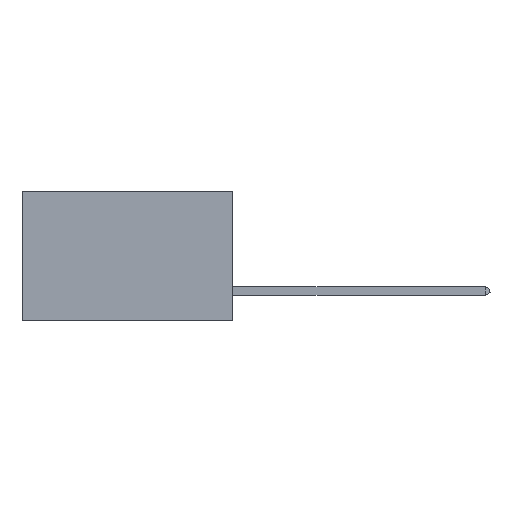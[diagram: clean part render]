
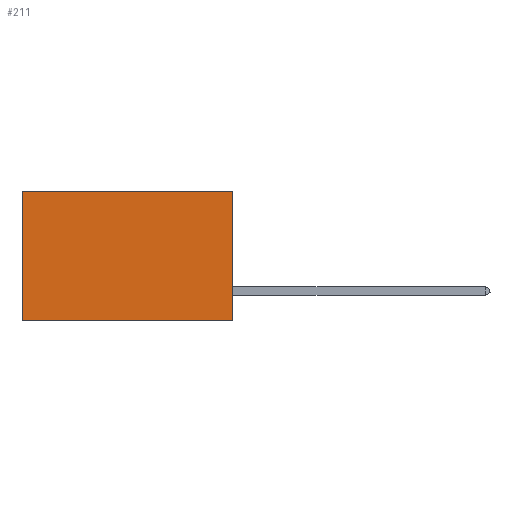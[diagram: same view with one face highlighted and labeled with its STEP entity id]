
A CAD part, left-side view. The second image highlights one B-rep face of the part: STEP entity #211.
In plain terms, the highlighted planar face has unit normal (-1, 0, 0).
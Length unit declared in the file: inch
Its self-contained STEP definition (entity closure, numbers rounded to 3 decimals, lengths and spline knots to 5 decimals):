
#211 = ADVANCED_FACE ( 'NONE', ( #1628 ), #21294, .F. ) ;
#1340 = LINE ( 'NONE', #2853, #17622 ) ;
#1628 = FACE_OUTER_BOUND ( 'NONE', #4700, .T. ) ;
#2272 = CARTESIAN_POINT ( 'NONE',  ( 0.2875, 0.6, -0.37 ) ) ;
#2853 = CARTESIAN_POINT ( 'NONE',  ( 0.2875, 0., -0.37 ) ) ;
#3857 = LINE ( 'NONE', #15583, #5583 ) ;
#4700 = EDGE_LOOP ( 'NONE', ( #33198, #25238, #16549, #34991 ) ) ;
#5583 = VECTOR ( 'NONE', #9802, 39.37008 ) ;
#6875 = DIRECTION ( 'NONE',  ( 0., 0., -1. ) ) ;
#7304 = LINE ( 'NONE', #31700, #45576 ) ;
#9411 = DIRECTION ( 'NONE',  ( 0., 0., -1. ) ) ;
#9802 = DIRECTION ( 'NONE',  ( 0., 0., -1. ) ) ;
#14392 = DIRECTION ( 'NONE',  ( 0., 1., 0. ) ) ;
#15583 = CARTESIAN_POINT ( 'NONE',  ( 0.2875, 0.6, 0. ) ) ;
#16549 = ORIENTED_EDGE ( 'NONE', *, *, #33871, .F. ) ;
#17622 = VECTOR ( 'NONE', #14392, 39.37008 ) ;
#21294 = PLANE ( 'NONE',  #31163 ) ;
#25238 = ORIENTED_EDGE ( 'NONE', *, *, #39706, .F. ) ;
#25338 = EDGE_CURVE ( 'NONE', #26952, #39386, #35256, .T. ) ;
#25958 = CARTESIAN_POINT ( 'NONE',  ( 0.2875, 0., 0. ) ) ;
#26176 = VERTEX_POINT ( 'NONE', #2272 ) ;
#26556 = EDGE_CURVE ( 'NONE', #39386, #26176, #3857, .T. ) ;
#26952 = VERTEX_POINT ( 'NONE', #25958 ) ;
#27146 = VERTEX_POINT ( 'NONE', #45243 ) ;
#30349 = DIRECTION ( 'NONE',  ( 0., 1., 0. ) ) ;
#30517 = CARTESIAN_POINT ( 'NONE',  ( 0.2875, 0., 0. ) ) ;
#31163 = AXIS2_PLACEMENT_3D ( 'NONE', #35999, #47078, #6875 ) ;
#31700 = CARTESIAN_POINT ( 'NONE',  ( 0.2875, 0., 0. ) ) ;
#33198 = ORIENTED_EDGE ( 'NONE', *, *, #26556, .T. ) ;
#33871 = EDGE_CURVE ( 'NONE', #26952, #27146, #7304, .T. ) ;
#34991 = ORIENTED_EDGE ( 'NONE', *, *, #25338, .T. ) ;
#35256 = LINE ( 'NONE', #30517, #41647 ) ;
#35999 = CARTESIAN_POINT ( 'NONE',  ( 0.2875, 0., 0. ) ) ;
#38155 = CARTESIAN_POINT ( 'NONE',  ( 0.2875, 0.6, 0. ) ) ;
#39386 = VERTEX_POINT ( 'NONE', #38155 ) ;
#39706 = EDGE_CURVE ( 'NONE', #27146, #26176, #1340, .T. ) ;
#41647 = VECTOR ( 'NONE', #30349, 39.37008 ) ;
#45243 = CARTESIAN_POINT ( 'NONE',  ( 0.2875, 0., -0.37 ) ) ;
#45576 = VECTOR ( 'NONE', #9411, 39.37008 ) ;
#47078 = DIRECTION ( 'NONE',  ( 1., 0., 0. ) ) ;
